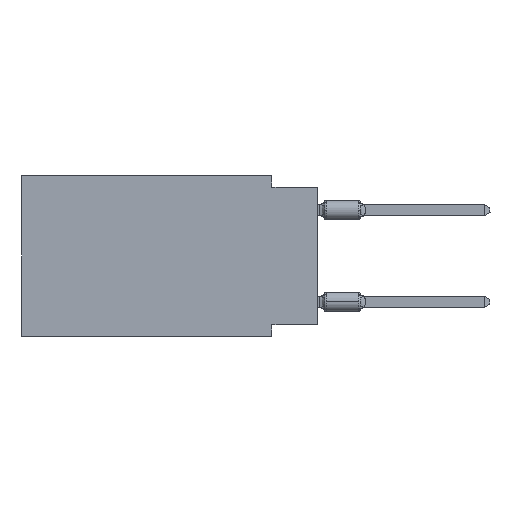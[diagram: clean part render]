
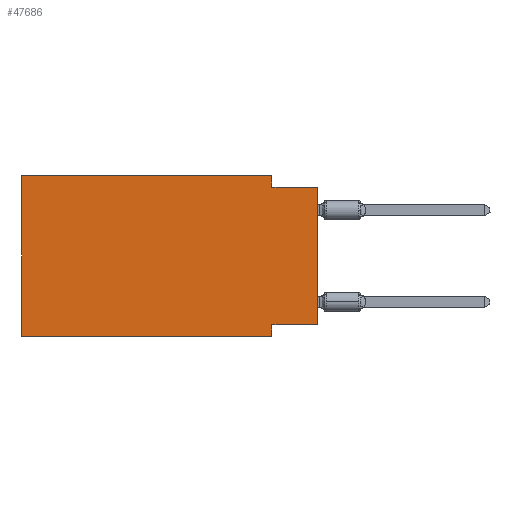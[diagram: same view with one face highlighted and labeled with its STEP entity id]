
A CAD part, left-side view. The second image highlights one B-rep face of the part: STEP entity #47686.
In plain terms, the highlighted planar face has unit normal (-1, 0, 0).
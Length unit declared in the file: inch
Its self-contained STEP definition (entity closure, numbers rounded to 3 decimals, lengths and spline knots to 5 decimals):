
#753 = VECTOR ( 'NONE', #16003, 39.37008 ) ;
#2627 = CARTESIAN_POINT ( 'NONE',  ( 0., 0.645, -0.35 ) ) ;
#3865 = DIRECTION ( 'NONE',  ( 0., 0., -1. ) ) ;
#5025 = EDGE_CURVE ( 'NONE', #32030, #25883, #56086, .T. ) ;
#5063 = EDGE_LOOP ( 'NONE', ( #69733, #43087, #16929, #5950, #60135, #59335, #7086, #42844 ) ) ;
#5326 = LINE ( 'NONE', #58137, #753 ) ;
#5950 = ORIENTED_EDGE ( 'NONE', *, *, #52441, .F. ) ;
#7052 = CARTESIAN_POINT ( 'NONE',  ( 0., 0.645, 0. ) ) ;
#7086 = ORIENTED_EDGE ( 'NONE', *, *, #61474, .F. ) ;
#7490 = VECTOR ( 'NONE', #29347, 39.37008 ) ;
#7794 = DIRECTION ( 'NONE',  ( 0., -1., 0. ) ) ;
#9242 = CARTESIAN_POINT ( 'NONE',  ( 0., 0., -0.325 ) ) ;
#10409 = CARTESIAN_POINT ( 'NONE',  ( 0., 0.645, 0. ) ) ;
#12069 = VECTOR ( 'NONE', #36976, 39.37008 ) ;
#13656 = CARTESIAN_POINT ( 'NONE',  ( 0., 0., -0.325 ) ) ;
#15044 = CARTESIAN_POINT ( 'NONE',  ( 0., 0.1, -0.025 ) ) ;
#16003 = DIRECTION ( 'NONE',  ( 0., 0., 1. ) ) ;
#16929 = ORIENTED_EDGE ( 'NONE', *, *, #27729, .F. ) ;
#17248 = VECTOR ( 'NONE', #59291, 39.37008 ) ;
#18133 = AXIS2_PLACEMENT_3D ( 'NONE', #67918, #57939, #63619 ) ;
#18137 = CARTESIAN_POINT ( 'NONE',  ( 0., 0.645, -0.35 ) ) ;
#19415 = PLANE ( 'NONE',  #18133 ) ;
#20617 = LINE ( 'NONE', #37406, #61843 ) ;
#20942 = EDGE_CURVE ( 'NONE', #32030, #27485, #5326, .T. ) ;
#25883 = VERTEX_POINT ( 'NONE', #33131 ) ;
#27199 = LINE ( 'NONE', #10409, #17248 ) ;
#27485 = VERTEX_POINT ( 'NONE', #49907 ) ;
#27729 = EDGE_CURVE ( 'NONE', #48789, #68339, #57713, .T. ) ;
#29347 = DIRECTION ( 'NONE',  ( 0., 1., 0. ) ) ;
#30966 = EDGE_CURVE ( 'NONE', #37484, #37699, #57333, .T. ) ;
#32030 = VERTEX_POINT ( 'NONE', #13656 ) ;
#33131 = CARTESIAN_POINT ( 'NONE',  ( 0., 0.1, -0.325 ) ) ;
#34051 = CARTESIAN_POINT ( 'NONE',  ( 0., 0., -0.025 ) ) ;
#34199 = LINE ( 'NONE', #60274, #60920 ) ;
#34308 = VERTEX_POINT ( 'NONE', #7052 ) ;
#36976 = DIRECTION ( 'NONE',  ( 0., 0., -1. ) ) ;
#37406 = CARTESIAN_POINT ( 'NONE',  ( 0., 0.1, -0.35 ) ) ;
#37484 = VERTEX_POINT ( 'NONE', #2627 ) ;
#37699 = VERTEX_POINT ( 'NONE', #55382 ) ;
#41275 = CARTESIAN_POINT ( 'NONE',  ( 0., 0.1, 0. ) ) ;
#41609 = VECTOR ( 'NONE', #49380, 39.37008 ) ;
#42844 = ORIENTED_EDGE ( 'NONE', *, *, #5025, .F. ) ;
#43087 = ORIENTED_EDGE ( 'NONE', *, *, #66944, .F. ) ;
#44411 = LINE ( 'NONE', #34051, #41609 ) ;
#44727 = CARTESIAN_POINT ( 'NONE',  ( 0., 0.1, 0. ) ) ;
#47686 = ADVANCED_FACE ( 'NONE', ( #52908 ), #19415, .F. ) ;
#48789 = VERTEX_POINT ( 'NONE', #44727 ) ;
#49380 = DIRECTION ( 'NONE',  ( 0., -1., 0. ) ) ;
#49907 = CARTESIAN_POINT ( 'NONE',  ( 0., 0., -0.025 ) ) ;
#50606 = DIRECTION ( 'NONE',  ( 0., 0., 1. ) ) ;
#52441 = EDGE_CURVE ( 'NONE', #34308, #48789, #27199, .T. ) ;
#52908 = FACE_OUTER_BOUND ( 'NONE', #5063, .T. ) ;
#55382 = CARTESIAN_POINT ( 'NONE',  ( 0., 0.1, -0.35 ) ) ;
#56086 = LINE ( 'NONE', #9242, #7490 ) ;
#57333 = LINE ( 'NONE', #18137, #61366 ) ;
#57713 = LINE ( 'NONE', #41275, #12069 ) ;
#57939 = DIRECTION ( 'NONE',  ( 1., 0., 0. ) ) ;
#58137 = CARTESIAN_POINT ( 'NONE',  ( 0., 0., 0. ) ) ;
#59291 = DIRECTION ( 'NONE',  ( 0., -1., 0. ) ) ;
#59335 = ORIENTED_EDGE ( 'NONE', *, *, #30966, .T. ) ;
#60135 = ORIENTED_EDGE ( 'NONE', *, *, #64863, .F. ) ;
#60274 = CARTESIAN_POINT ( 'NONE',  ( 0., 0.645, 0. ) ) ;
#60920 = VECTOR ( 'NONE', #50606, 39.37008 ) ;
#61366 = VECTOR ( 'NONE', #7794, 39.37008 ) ;
#61474 = EDGE_CURVE ( 'NONE', #25883, #37699, #20617, .T. ) ;
#61843 = VECTOR ( 'NONE', #3865, 39.37008 ) ;
#63619 = DIRECTION ( 'NONE',  ( 0., 0., -1. ) ) ;
#64863 = EDGE_CURVE ( 'NONE', #37484, #34308, #34199, .T. ) ;
#66944 = EDGE_CURVE ( 'NONE', #68339, #27485, #44411, .T. ) ;
#67918 = CARTESIAN_POINT ( 'NONE',  ( 0., 0.645, 0. ) ) ;
#68339 = VERTEX_POINT ( 'NONE', #15044 ) ;
#69733 = ORIENTED_EDGE ( 'NONE', *, *, #20942, .T. ) ;
